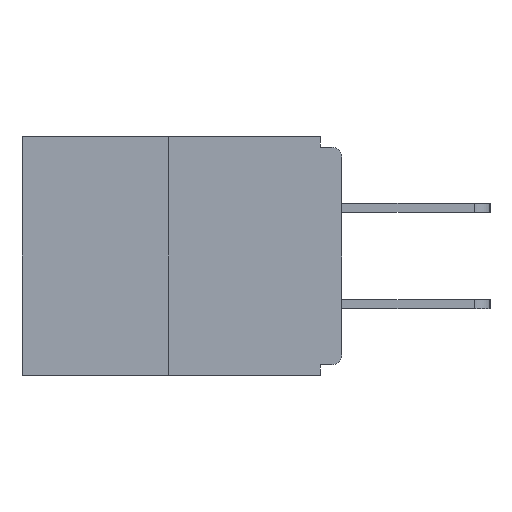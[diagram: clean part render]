
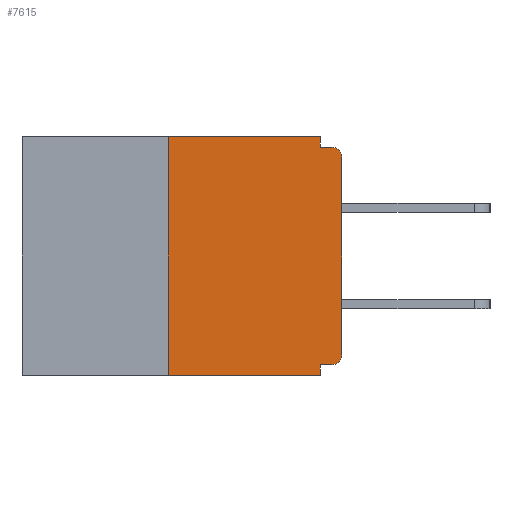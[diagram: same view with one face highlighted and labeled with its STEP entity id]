
A CAD part, left-side view. The second image highlights one B-rep face of the part: STEP entity #7615.
In plain terms, the highlighted planar face has unit normal (-1, 0, 0).
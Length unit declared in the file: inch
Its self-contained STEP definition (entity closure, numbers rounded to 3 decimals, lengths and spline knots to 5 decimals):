
#111 = VERTEX_POINT ( 'NONE', #5924 ) ;
#483 = CARTESIAN_POINT ( 'NONE',  ( 0., 0.46, -0.343 ) ) ;
#749 = VECTOR ( 'NONE', #9329, 39.37008 ) ;
#1074 = EDGE_CURVE ( 'NONE', #4633, #24947, #9184, .T. ) ;
#1282 = ORIENTED_EDGE ( 'NONE', *, *, #1074, .F. ) ;
#1568 = EDGE_CURVE ( 'NONE', #5504, #19948, #17139, .T. ) ;
#1997 = CARTESIAN_POINT ( 'NONE',  ( 0., 0., -0.015 ) ) ;
#2169 = VECTOR ( 'NONE', #7044, 39.37008 ) ;
#2329 = CARTESIAN_POINT ( 'NONE',  ( 0., 0.25, 0. ) ) ;
#3205 = LINE ( 'NONE', #483, #16221 ) ;
#3510 = CARTESIAN_POINT ( 'NONE',  ( 0., 0.015, -0.328 ) ) ;
#3800 = CIRCLE ( 'NONE', #9484, 0.015 ) ;
#4041 = CARTESIAN_POINT ( 'NONE',  ( 0., 0.015, -0.313 ) ) ;
#4287 = VERTEX_POINT ( 'NONE', #13302 ) ;
#4297 = CARTESIAN_POINT ( 'NONE',  ( 0., 0.25, -0.343 ) ) ;
#4633 = VERTEX_POINT ( 'NONE', #26171 ) ;
#5504 = VERTEX_POINT ( 'NONE', #4297 ) ;
#5924 = CARTESIAN_POINT ( 'NONE',  ( 0., 0.031, -0.328 ) ) ;
#6260 = DIRECTION ( 'NONE',  ( 0., 1., 0. ) ) ;
#7033 = VECTOR ( 'NONE', #6260, 39.37008 ) ;
#7044 = DIRECTION ( 'NONE',  ( 0., 0., 1. ) ) ;
#7228 = VERTEX_POINT ( 'NONE', #3510 ) ;
#7423 = DIRECTION ( 'NONE',  ( 1., 0., 0. ) ) ;
#7615 = ADVANCED_FACE ( 'NONE', ( #23362 ), #7697, .F. ) ;
#7697 = PLANE ( 'NONE',  #19540 ) ;
#8221 = DIRECTION ( 'NONE',  ( 0., 0., -1. ) ) ;
#8269 = DIRECTION ( 'NONE',  ( 0., -1., 0. ) ) ;
#8414 = ORIENTED_EDGE ( 'NONE', *, *, #20284, .T. ) ;
#8646 = ORIENTED_EDGE ( 'NONE', *, *, #23330, .F. ) ;
#8773 = VECTOR ( 'NONE', #13236, 39.37008 ) ;
#8843 = CARTESIAN_POINT ( 'NONE',  ( 0., 0.25, 0. ) ) ;
#9184 = LINE ( 'NONE', #1997, #22882 ) ;
#9329 = DIRECTION ( 'NONE',  ( 0., 0., -1. ) ) ;
#9342 = CARTESIAN_POINT ( 'NONE',  ( 0., 0.015, -0.03 ) ) ;
#9484 = AXIS2_PLACEMENT_3D ( 'NONE', #9342, #23566, #11395 ) ;
#10138 = ORIENTED_EDGE ( 'NONE', *, *, #22796, .F. ) ;
#10879 = CARTESIAN_POINT ( 'NONE',  ( 0., 0.031, 0. ) ) ;
#10925 = ORIENTED_EDGE ( 'NONE', *, *, #1568, .F. ) ;
#11395 = DIRECTION ( 'NONE',  ( 0., 0., -1. ) ) ;
#11748 = VERTEX_POINT ( 'NONE', #10879 ) ;
#13236 = DIRECTION ( 'NONE',  ( 0., 0., 1. ) ) ;
#13302 = CARTESIAN_POINT ( 'NONE',  ( 0., 0., -0.03 ) ) ;
#14188 = DIRECTION ( 'NONE',  ( -1., 0., 0. ) ) ;
#14505 = EDGE_CURVE ( 'NONE', #5504, #14640, #3205, .T. ) ;
#14549 = DIRECTION ( 'NONE',  ( 0., -1., 0. ) ) ;
#14640 = VERTEX_POINT ( 'NONE', #21048 ) ;
#15199 = CARTESIAN_POINT ( 'NONE',  ( 0., 0., 0. ) ) ;
#15273 = DIRECTION ( 'NONE',  ( 0., -1., 0. ) ) ;
#15318 = ORIENTED_EDGE ( 'NONE', *, *, #16628, .T. ) ;
#15889 = CARTESIAN_POINT ( 'NONE',  ( 0., 0.46, 0. ) ) ;
#16221 = VECTOR ( 'NONE', #14549, 39.37008 ) ;
#16628 = EDGE_CURVE ( 'NONE', #25561, #4287, #16745, .T. ) ;
#16718 = AXIS2_PLACEMENT_3D ( 'NONE', #4041, #14188, #20234 ) ;
#16745 = LINE ( 'NONE', #15199, #8773 ) ;
#17139 = LINE ( 'NONE', #8843, #2169 ) ;
#17270 = LINE ( 'NONE', #23375, #21395 ) ;
#17573 = EDGE_CURVE ( 'NONE', #11748, #4633, #25276, .T. ) ;
#17746 = ORIENTED_EDGE ( 'NONE', *, *, #24849, .T. ) ;
#17970 = CARTESIAN_POINT ( 'NONE',  ( 0., 0.015, -0.015 ) ) ;
#18719 = CARTESIAN_POINT ( 'NONE',  ( 0., 0., -0.328 ) ) ;
#19540 = AXIS2_PLACEMENT_3D ( 'NONE', #15889, #7423, #19982 ) ;
#19948 = VERTEX_POINT ( 'NONE', #2329 ) ;
#19982 = DIRECTION ( 'NONE',  ( 0., 0., -1. ) ) ;
#20234 = DIRECTION ( 'NONE',  ( 0., 0., -1. ) ) ;
#20284 = EDGE_CURVE ( 'NONE', #7228, #25561, #21284, .T. ) ;
#20405 = ORIENTED_EDGE ( 'NONE', *, *, #17573, .F. ) ;
#20437 = CARTESIAN_POINT ( 'NONE',  ( 0., 0.031, 0. ) ) ;
#21048 = CARTESIAN_POINT ( 'NONE',  ( 0., 0.031, -0.343 ) ) ;
#21284 = CIRCLE ( 'NONE', #16718, 0.015 ) ;
#21335 = CARTESIAN_POINT ( 'NONE',  ( 0., 0., -0.313 ) ) ;
#21395 = VECTOR ( 'NONE', #15273, 39.37008 ) ;
#21522 = CARTESIAN_POINT ( 'NONE',  ( 0., 0.031, -0.343 ) ) ;
#22347 = ORIENTED_EDGE ( 'NONE', *, *, #23078, .F. ) ;
#22796 = EDGE_CURVE ( 'NONE', #111, #14640, #23038, .T. ) ;
#22882 = VECTOR ( 'NONE', #8269, 39.37008 ) ;
#23038 = LINE ( 'NONE', #21522, #749 ) ;
#23056 = VECTOR ( 'NONE', #8221, 39.37008 ) ;
#23078 = EDGE_CURVE ( 'NONE', #19948, #11748, #17270, .T. ) ;
#23267 = LINE ( 'NONE', #18719, #7033 ) ;
#23330 = EDGE_CURVE ( 'NONE', #7228, #111, #23267, .T. ) ;
#23362 = FACE_OUTER_BOUND ( 'NONE', #23749, .T. ) ;
#23375 = CARTESIAN_POINT ( 'NONE',  ( 0., 0.46, 0. ) ) ;
#23566 = DIRECTION ( 'NONE',  ( -1., 0., 0. ) ) ;
#23749 = EDGE_LOOP ( 'NONE', ( #22347, #10925, #24820, #10138, #8646, #8414, #15318, #17746, #1282, #20405 ) ) ;
#24820 = ORIENTED_EDGE ( 'NONE', *, *, #14505, .T. ) ;
#24849 = EDGE_CURVE ( 'NONE', #4287, #24947, #3800, .T. ) ;
#24947 = VERTEX_POINT ( 'NONE', #17970 ) ;
#25276 = LINE ( 'NONE', #20437, #23056 ) ;
#25561 = VERTEX_POINT ( 'NONE', #21335 ) ;
#26171 = CARTESIAN_POINT ( 'NONE',  ( 0., 0.031, -0.015 ) ) ;
